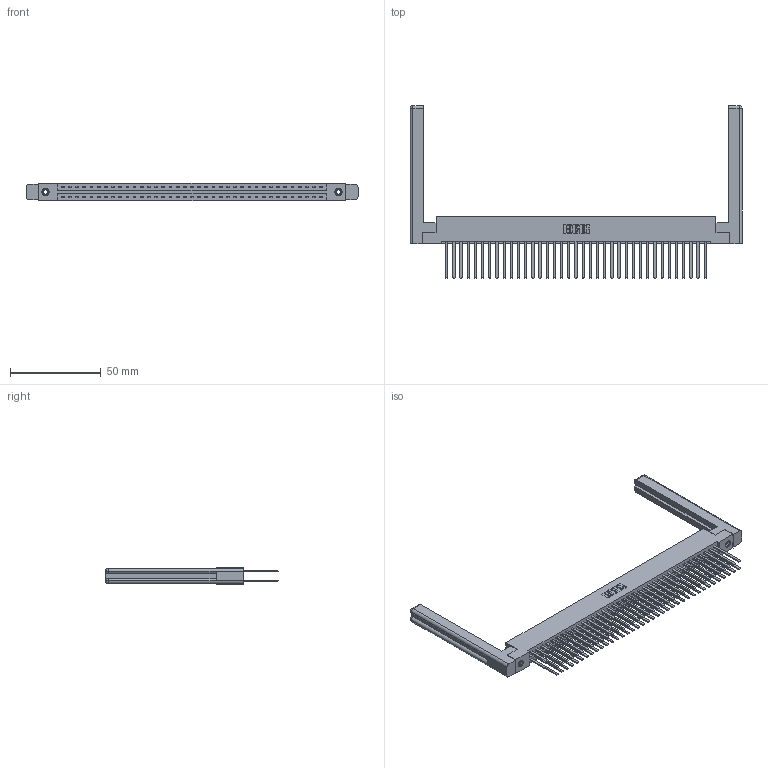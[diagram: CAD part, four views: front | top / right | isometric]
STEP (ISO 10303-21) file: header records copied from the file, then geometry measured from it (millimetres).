
FILE_DESCRIPTION (( 'STEP AP203' ), '1' );
FILE_NAME ('337-074-544-258.STEP', '2019-10-10T04:03:00', ( '' ), ( '' ), 'SwSTEP 2.0', 'SolidWorks 2016', '' );
FILE_SCHEMA (( 'CONFIG_CONTROL_DESIGN' ));
Length unit declared in the file: inch
Products named in the file (5): 337 Part_Flush Mounting Lugs - 0.156 Dia-TI; 345-292-001_345-293-144; 337-074-544-258; 345-250-001_345-250-001-102; 307-220-058
Assembly tree (79 placements, depth 2):
  337-074-544-258
    337 Part_Flush Mounting Lugs - 0.156 Dia-TI
    345-292-001_345-293-144  x74
    345-250-001_345-250-001-102  x2
    307-220-058  x2
Bounding box: 183.24 x 95.38 x 9.4 mm (x, y, z)
Volume: 27424 mm3; surface area: 31315.3 mm2
Topology: 79 solids, 79 shells, 3808 faces, 11247 edges, 7386 vertices
Faces by surface type: plane 2670, cylinder 1114, cone 12, torus 12
Entity records: 31784 total; most frequent: CARTESIAN_POINT 5365, ORIENTED_EDGE 5240, DIRECTION 4584, EDGE_CURVE 2620, LINE 2448, VECTOR 2448, VERTEX_POINT 1738, AXIS2_PLACEMENT_3D 1068
